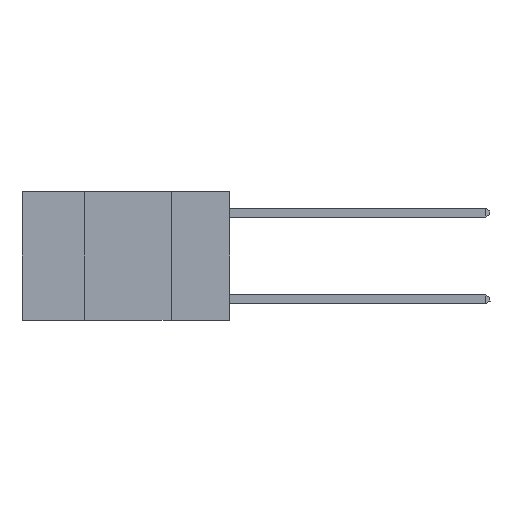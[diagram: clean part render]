
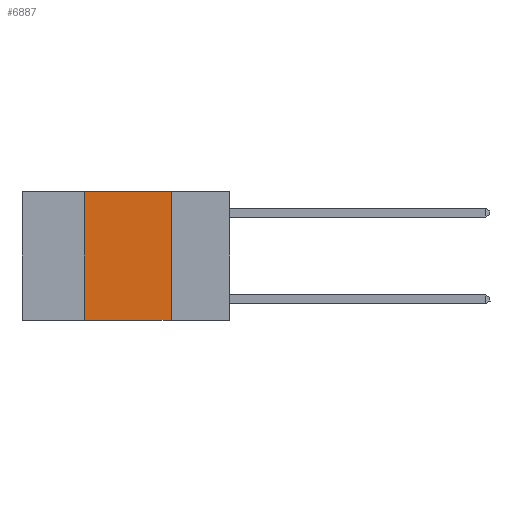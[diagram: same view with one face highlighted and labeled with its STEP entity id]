
A CAD part, left-side view. The second image highlights one B-rep face of the part: STEP entity #6887.
In plain terms, the highlighted planar face has unit normal (-1, 0, 0).
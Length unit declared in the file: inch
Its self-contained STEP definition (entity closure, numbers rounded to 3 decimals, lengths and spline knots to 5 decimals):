
#580 = CARTESIAN_POINT ( 'NONE',  ( 0., 0.42, 0. ) ) ;
#938 = DIRECTION ( 'NONE',  ( 0., 0., -1. ) ) ;
#1162 = ORIENTED_EDGE ( 'NONE', *, *, #1644, .F. ) ;
#1644 = EDGE_CURVE ( 'NONE', #19913, #9523, #8828, .T. ) ;
#2127 = VERTEX_POINT ( 'NONE', #14329 ) ;
#2828 = EDGE_CURVE ( 'NONE', #2127, #7921, #5015, .T. ) ;
#5015 = LINE ( 'NONE', #12504, #13916 ) ;
#6887 = ADVANCED_FACE ( 'NONE', ( #11764 ), #7956, .F. ) ;
#7105 = ORIENTED_EDGE ( 'NONE', *, *, #2828, .F. ) ;
#7137 = CARTESIAN_POINT ( 'NONE',  ( 0., 0.17, -0.37 ) ) ;
#7308 = VECTOR ( 'NONE', #12685, 39.37008 ) ;
#7483 = AXIS2_PLACEMENT_3D ( 'NONE', #20498, #11562, #938 ) ;
#7921 = VERTEX_POINT ( 'NONE', #7137 ) ;
#7956 = PLANE ( 'NONE',  #7483 ) ;
#8658 = CARTESIAN_POINT ( 'NONE',  ( 0., 0.42, 0. ) ) ;
#8828 = LINE ( 'NONE', #8658, #18386 ) ;
#9523 = VERTEX_POINT ( 'NONE', #580 ) ;
#10121 = EDGE_LOOP ( 'NONE', ( #7105, #19294, #1162, #18444 ) ) ;
#11562 = DIRECTION ( 'NONE',  ( 1., 0., 0. ) ) ;
#11700 = CARTESIAN_POINT ( 'NONE',  ( 0., 0.6, 0. ) ) ;
#11764 = FACE_OUTER_BOUND ( 'NONE', #10121, .T. ) ;
#12504 = CARTESIAN_POINT ( 'NONE',  ( 0., 0.17, 0. ) ) ;
#12685 = DIRECTION ( 'NONE',  ( 0., -1., 0. ) ) ;
#12766 = EDGE_CURVE ( 'NONE', #9523, #2127, #21087, .T. ) ;
#13392 = CARTESIAN_POINT ( 'NONE',  ( 0., 0.42, -0.37 ) ) ;
#13916 = VECTOR ( 'NONE', #14307, 39.37008 ) ;
#14307 = DIRECTION ( 'NONE',  ( 0., 0., -1. ) ) ;
#14329 = CARTESIAN_POINT ( 'NONE',  ( 0., 0.17, 0. ) ) ;
#15780 = VECTOR ( 'NONE', #20643, 39.37008 ) ;
#16871 = EDGE_CURVE ( 'NONE', #19913, #7921, #21586, .T. ) ;
#18386 = VECTOR ( 'NONE', #19647, 39.37008 ) ;
#18444 = ORIENTED_EDGE ( 'NONE', *, *, #16871, .T. ) ;
#19294 = ORIENTED_EDGE ( 'NONE', *, *, #12766, .F. ) ;
#19647 = DIRECTION ( 'NONE',  ( 0., 0., 1. ) ) ;
#19913 = VERTEX_POINT ( 'NONE', #13392 ) ;
#20498 = CARTESIAN_POINT ( 'NONE',  ( 0., 0.6, 0. ) ) ;
#20643 = DIRECTION ( 'NONE',  ( 0., -1., 0. ) ) ;
#21087 = LINE ( 'NONE', #11700, #15780 ) ;
#21543 = CARTESIAN_POINT ( 'NONE',  ( 0., 0.6, -0.37 ) ) ;
#21586 = LINE ( 'NONE', #21543, #7308 ) ;
